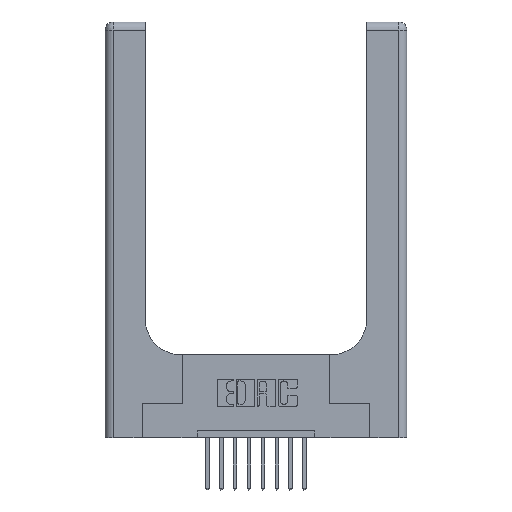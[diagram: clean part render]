
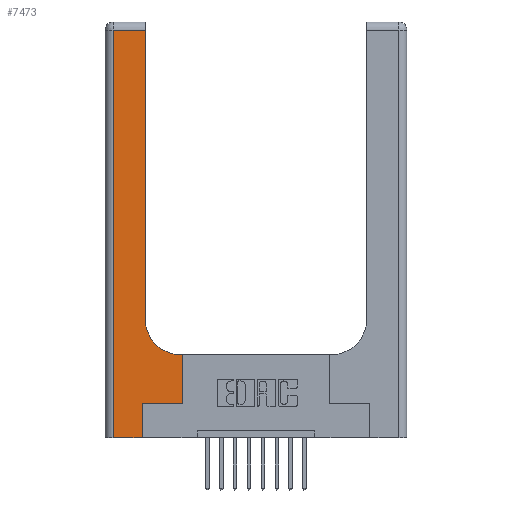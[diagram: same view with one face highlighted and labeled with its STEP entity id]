
A CAD part, top view. The second image highlights one B-rep face of the part: STEP entity #7473.
In plain terms, the highlighted planar face has unit normal (0, 0, 1).
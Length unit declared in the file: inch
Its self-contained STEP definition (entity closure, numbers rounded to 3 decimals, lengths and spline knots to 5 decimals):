
#33 = VECTOR ( 'NONE', #223, 39.37008 ) ;
#223 = DIRECTION ( 'NONE',  ( -1., 0., 0. ) ) ;
#236 = CARTESIAN_POINT ( 'NONE',  ( 0.269, 0.25, 0.37 ) ) ;
#286 = LINE ( 'NONE', #8022, #13281 ) ;
#394 = ORIENTED_EDGE ( 'NONE', *, *, #13972, .T. ) ;
#553 = LINE ( 'NONE', #13918, #5693 ) ;
#697 = ORIENTED_EDGE ( 'NONE', *, *, #2601, .T. ) ;
#835 = DIRECTION ( 'NONE',  ( 0., 0., -1. ) ) ;
#896 = LINE ( 'NONE', #4577, #15576 ) ;
#1087 = ORIENTED_EDGE ( 'NONE', *, *, #12852, .T. ) ;
#1363 = CARTESIAN_POINT ( 'NONE',  ( 0.2915, 0.6, 0.37 ) ) ;
#1509 = CARTESIAN_POINT ( 'NONE',  ( 0.2915, 3., 0.37 ) ) ;
#1637 = DIRECTION ( 'NONE',  ( 0., 0., -1. ) ) ;
#1665 = EDGE_CURVE ( 'NONE', #9807, #15105, #553, .T. ) ;
#2026 = DIRECTION ( 'NONE',  ( 1., 0., 0. ) ) ;
#2088 = EDGE_CURVE ( 'NONE', #2562, #5682, #8552, .T. ) ;
#2171 = VECTOR ( 'NONE', #10308, 39.37008 ) ;
#2562 = VERTEX_POINT ( 'NONE', #5399 ) ;
#2601 = EDGE_CURVE ( 'NONE', #3932, #4817, #9631, .T. ) ;
#2626 = EDGE_CURVE ( 'NONE', #9668, #3932, #286, .T. ) ;
#2645 = LINE ( 'NONE', #1509, #10684 ) ;
#2719 = CARTESIAN_POINT ( 'NONE',  ( 0.2915, 2.94, 0.37 ) ) ;
#2920 = ORIENTED_EDGE ( 'NONE', *, *, #3512, .T. ) ;
#3512 = EDGE_CURVE ( 'NONE', #10971, #8723, #8457, .T. ) ;
#3727 = CARTESIAN_POINT ( 'NONE',  ( 0.06, 0., 0.37 ) ) ;
#3924 = DIRECTION ( 'NONE',  ( 0., 1., 0. ) ) ;
#3932 = VERTEX_POINT ( 'NONE', #11282 ) ;
#3985 = ORIENTED_EDGE ( 'NONE', *, *, #15579, .T. ) ;
#4421 = CARTESIAN_POINT ( 'NONE',  ( 0.5585, 0.6, 0.37 ) ) ;
#4577 = CARTESIAN_POINT ( 'NONE',  ( 0.06, 3., 0.37 ) ) ;
#4817 = VERTEX_POINT ( 'NONE', #7834 ) ;
#5210 = VECTOR ( 'NONE', #14840, 39.37008 ) ;
#5399 = CARTESIAN_POINT ( 'NONE',  ( 0.5415, 0.6, 0.37 ) ) ;
#5530 = AXIS2_PLACEMENT_3D ( 'NONE', #12781, #1637, #10158 ) ;
#5682 = VERTEX_POINT ( 'NONE', #11977 ) ;
#5693 = VECTOR ( 'NONE', #6513, 39.37008 ) ;
#6098 = LINE ( 'NONE', #236, #15663 ) ;
#6121 = ORIENTED_EDGE ( 'NONE', *, *, #11847, .T. ) ;
#6513 = DIRECTION ( 'NONE',  ( -1., 0., 0. ) ) ;
#6887 = CARTESIAN_POINT ( 'NONE',  ( 0.5415, 0.85, 0.37 ) ) ;
#7473 = ADVANCED_FACE ( 'NONE', ( #8517 ), #14035, .F. ) ;
#7543 = ORIENTED_EDGE ( 'NONE', *, *, #2088, .T. ) ;
#7834 = CARTESIAN_POINT ( 'NONE',  ( 0.269, 0.25, 0.37 ) ) ;
#7858 = CARTESIAN_POINT ( 'NONE',  ( 0.269, 0., 0.37 ) ) ;
#8022 = CARTESIAN_POINT ( 'NONE',  ( 0., 0., 0.37 ) ) ;
#8041 = DIRECTION ( 'NONE',  ( 1., 0., 0. ) ) ;
#8102 = ORIENTED_EDGE ( 'NONE', *, *, #1665, .T. ) ;
#8457 = LINE ( 'NONE', #9529, #5210 ) ;
#8517 = FACE_OUTER_BOUND ( 'NONE', #11810, .T. ) ;
#8552 = CIRCLE ( 'NONE', #12157, 0.25 ) ;
#8723 = VERTEX_POINT ( 'NONE', #4421 ) ;
#9529 = CARTESIAN_POINT ( 'NONE',  ( 0.5585, 0.25, 0.37 ) ) ;
#9631 = LINE ( 'NONE', #7858, #2171 ) ;
#9668 = VERTEX_POINT ( 'NONE', #3727 ) ;
#9777 = LINE ( 'NONE', #1363, #33 ) ;
#9807 = VERTEX_POINT ( 'NONE', #2719 ) ;
#10158 = DIRECTION ( 'NONE',  ( -1., 0., 0. ) ) ;
#10308 = DIRECTION ( 'NONE',  ( 0., 1., 0. ) ) ;
#10684 = VECTOR ( 'NONE', #3924, 39.37008 ) ;
#10971 = VERTEX_POINT ( 'NONE', #11654 ) ;
#11282 = CARTESIAN_POINT ( 'NONE',  ( 0.269, 0., 0.37 ) ) ;
#11654 = CARTESIAN_POINT ( 'NONE',  ( 0.5585, 0.25, 0.37 ) ) ;
#11810 = EDGE_LOOP ( 'NONE', ( #394, #8102, #3985, #15278, #697, #1087, #2920, #6121, #7543 ) ) ;
#11847 = EDGE_CURVE ( 'NONE', #8723, #2562, #9777, .T. ) ;
#11977 = CARTESIAN_POINT ( 'NONE',  ( 0.2915, 0.85, 0.37 ) ) ;
#12157 = AXIS2_PLACEMENT_3D ( 'NONE', #6887, #835, #8041 ) ;
#12781 = CARTESIAN_POINT ( 'NONE',  ( 0., 3., 0.37 ) ) ;
#12852 = EDGE_CURVE ( 'NONE', #4817, #10971, #6098, .T. ) ;
#13281 = VECTOR ( 'NONE', #2026, 39.37008 ) ;
#13498 = DIRECTION ( 'NONE',  ( 1., 0., 0. ) ) ;
#13918 = CARTESIAN_POINT ( 'NONE',  ( 0., 2.94, 0.37 ) ) ;
#13972 = EDGE_CURVE ( 'NONE', #5682, #9807, #2645, .T. ) ;
#14035 = PLANE ( 'NONE',  #5530 ) ;
#14606 = CARTESIAN_POINT ( 'NONE',  ( 0.06, 2.94, 0.37 ) ) ;
#14840 = DIRECTION ( 'NONE',  ( 0., 1., 0. ) ) ;
#15105 = VERTEX_POINT ( 'NONE', #14606 ) ;
#15278 = ORIENTED_EDGE ( 'NONE', *, *, #2626, .T. ) ;
#15533 = DIRECTION ( 'NONE',  ( 0., -1., 0. ) ) ;
#15576 = VECTOR ( 'NONE', #15533, 39.37008 ) ;
#15579 = EDGE_CURVE ( 'NONE', #15105, #9668, #896, .T. ) ;
#15663 = VECTOR ( 'NONE', #13498, 39.37008 ) ;
